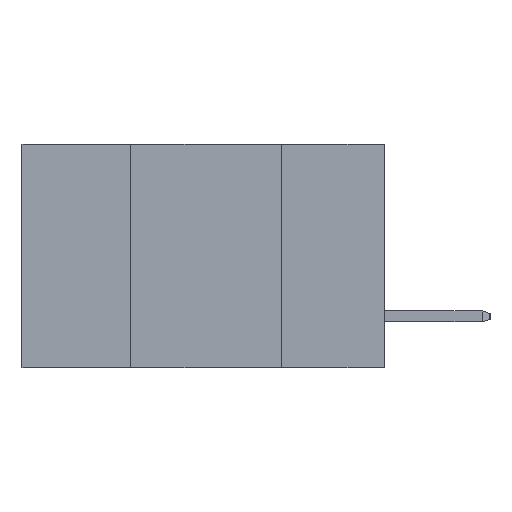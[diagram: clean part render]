
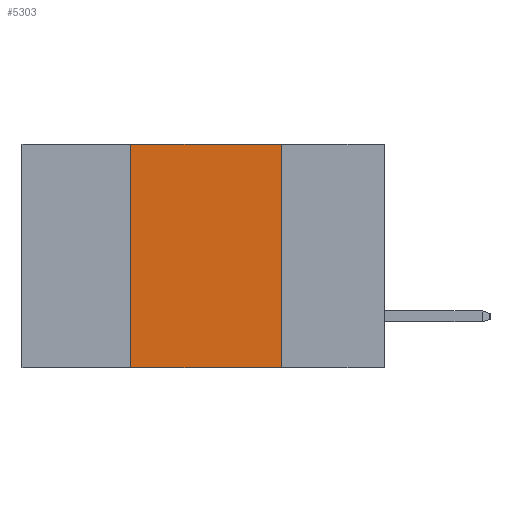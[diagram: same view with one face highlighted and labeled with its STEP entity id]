
A CAD part, left-side view. The second image highlights one B-rep face of the part: STEP entity #5303.
In plain terms, the highlighted planar face has unit normal (-1, 0, 0).
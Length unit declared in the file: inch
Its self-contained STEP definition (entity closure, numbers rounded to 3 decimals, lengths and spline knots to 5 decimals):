
#182 = CARTESIAN_POINT ( 'NONE',  ( 0., 0.6, 0. ) ) ;
#495 = VECTOR ( 'NONE', #4351, 39.37008 ) ;
#1268 = ORIENTED_EDGE ( 'NONE', *, *, #3511, .T. ) ;
#1280 = LINE ( 'NONE', #182, #4406 ) ;
#1288 = EDGE_CURVE ( 'NONE', #7308, #3909, #5695, .T. ) ;
#1405 = CARTESIAN_POINT ( 'NONE',  ( 0., 0.42, -0.37 ) ) ;
#1571 = CARTESIAN_POINT ( 'NONE',  ( 0., 0.42, -0.37 ) ) ;
#1590 = DIRECTION ( 'NONE',  ( 1., 0., 0. ) ) ;
#1615 = DIRECTION ( 'NONE',  ( 0., 0., -1. ) ) ;
#2280 = DIRECTION ( 'NONE',  ( 0., -1., 0. ) ) ;
#2416 = CARTESIAN_POINT ( 'NONE',  ( 0., 0.17, -0.37 ) ) ;
#2669 = DIRECTION ( 'NONE',  ( 0., -1., 0. ) ) ;
#2712 = CARTESIAN_POINT ( 'NONE',  ( 0., 0.6, -0.37 ) ) ;
#2963 = ORIENTED_EDGE ( 'NONE', *, *, #1288, .F. ) ;
#3161 = EDGE_LOOP ( 'NONE', ( #2963, #4065, #5283, #1268 ) ) ;
#3414 = VERTEX_POINT ( 'NONE', #1405 ) ;
#3511 = EDGE_CURVE ( 'NONE', #3414, #3909, #6882, .T. ) ;
#3909 = VERTEX_POINT ( 'NONE', #7148 ) ;
#4065 = ORIENTED_EDGE ( 'NONE', *, *, #7000, .F. ) ;
#4351 = DIRECTION ( 'NONE',  ( 0., 0., -1. ) ) ;
#4406 = VECTOR ( 'NONE', #2280, 39.37008 ) ;
#4874 = AXIS2_PLACEMENT_3D ( 'NONE', #4948, #1590, #1615 ) ;
#4948 = CARTESIAN_POINT ( 'NONE',  ( 0., 0.6, 0. ) ) ;
#5112 = VECTOR ( 'NONE', #2669, 39.37008 ) ;
#5230 = CARTESIAN_POINT ( 'NONE',  ( 0., 0.17, 0. ) ) ;
#5283 = ORIENTED_EDGE ( 'NONE', *, *, #8144, .F. ) ;
#5303 = ADVANCED_FACE ( 'NONE', ( #7703 ), #5660, .F. ) ;
#5364 = LINE ( 'NONE', #1571, #5580 ) ;
#5580 = VECTOR ( 'NONE', #5608, 39.37008 ) ;
#5608 = DIRECTION ( 'NONE',  ( 0., 0., 1. ) ) ;
#5660 = PLANE ( 'NONE',  #4874 ) ;
#5695 = LINE ( 'NONE', #2416, #495 ) ;
#6882 = LINE ( 'NONE', #2712, #5112 ) ;
#7000 = EDGE_CURVE ( 'NONE', #8505, #7308, #1280, .T. ) ;
#7148 = CARTESIAN_POINT ( 'NONE',  ( 0., 0.17, -0.37 ) ) ;
#7308 = VERTEX_POINT ( 'NONE', #5230 ) ;
#7316 = CARTESIAN_POINT ( 'NONE',  ( 0., 0.42, 0. ) ) ;
#7703 = FACE_OUTER_BOUND ( 'NONE', #3161, .T. ) ;
#8144 = EDGE_CURVE ( 'NONE', #3414, #8505, #5364, .T. ) ;
#8505 = VERTEX_POINT ( 'NONE', #7316 ) ;
